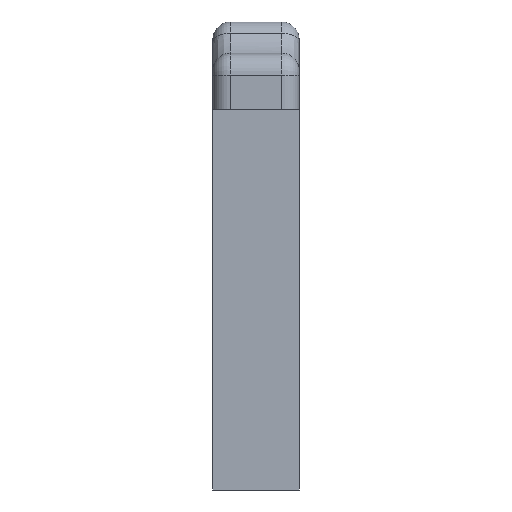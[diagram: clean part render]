
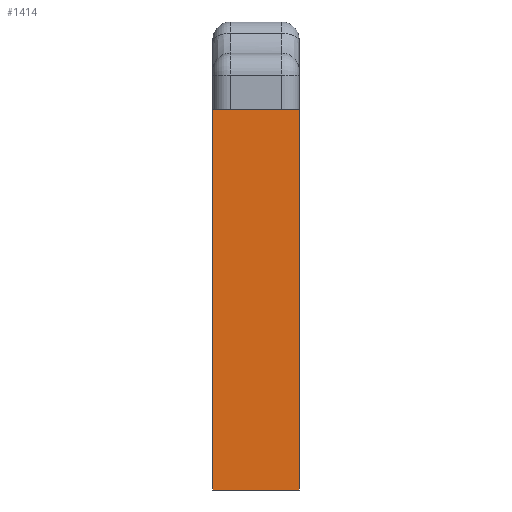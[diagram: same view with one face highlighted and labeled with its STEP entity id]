
A CAD part, front view. The second image highlights one B-rep face of the part: STEP entity #1414.
In plain terms, the highlighted planar face has unit normal (0, -1, 0).
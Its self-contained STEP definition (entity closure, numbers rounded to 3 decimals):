
#30 = EDGE_CURVE ( 'NONE', #1601, #479, #509, .T. ) ;
#61 = DIRECTION ( 'NONE',  ( -1., 0., 0. ) ) ;
#64 = CARTESIAN_POINT ( 'NONE',  ( 9.898, -2.5, -38.75 ) ) ;
#127 = ORIENTED_EDGE ( 'NONE', *, *, #1538, .T. ) ;
#147 = CARTESIAN_POINT ( 'NONE',  ( 9.898, -2.5, 5. ) ) ;
#215 = DIRECTION ( 'NONE',  ( 0., 0., 1. ) ) ;
#233 = DIRECTION ( 'NONE',  ( 0., 1., 0. ) ) ;
#237 = CARTESIAN_POINT ( 'NONE',  ( 9.898, -2.5, 15. ) ) ;
#337 = PLANE ( 'NONE',  #654 ) ;
#467 = VECTOR ( 'NONE', #1634, 1000. ) ;
#479 = VERTEX_POINT ( 'NONE', #823 ) ;
#486 = LINE ( 'NONE', #537, #467 ) ;
#488 = VECTOR ( 'NONE', #1300, 1000. ) ;
#505 = DIRECTION ( 'NONE',  ( 1., 0., 0. ) ) ;
#509 = LINE ( 'NONE', #1474, #488 ) ;
#514 = CARTESIAN_POINT ( 'NONE',  ( 9.898, -2.5, 5. ) ) ;
#529 = VERTEX_POINT ( 'NONE', #739 ) ;
#537 = CARTESIAN_POINT ( 'NONE',  ( 0., -2.5, 15. ) ) ;
#616 = FACE_OUTER_BOUND ( 'NONE', #986, .T. ) ;
#654 = AXIS2_PLACEMENT_3D ( 'NONE', #237, #233, #215 ) ;
#739 = CARTESIAN_POINT ( 'NONE',  ( 0., -2.5, 5. ) ) ;
#823 = CARTESIAN_POINT ( 'NONE',  ( 9.898, -2.5, -38.75 ) ) ;
#885 = EDGE_CURVE ( 'NONE', #479, #1052, #1165, .T. ) ;
#935 = VECTOR ( 'NONE', #505, 1000. ) ;
#957 = ORIENTED_EDGE ( 'NONE', *, *, #1108, .F. ) ;
#958 = LINE ( 'NONE', #147, #935 ) ;
#986 = EDGE_LOOP ( 'NONE', ( #957, #127, #1262, #1286 ) ) ;
#1052 = VERTEX_POINT ( 'NONE', #1321 ) ;
#1108 = EDGE_CURVE ( 'NONE', #529, #1601, #958, .T. ) ;
#1165 = LINE ( 'NONE', #64, #1182 ) ;
#1182 = VECTOR ( 'NONE', #61, 1000. ) ;
#1262 = ORIENTED_EDGE ( 'NONE', *, *, #885, .F. ) ;
#1286 = ORIENTED_EDGE ( 'NONE', *, *, #30, .F. ) ;
#1300 = DIRECTION ( 'NONE',  ( 0., 0., -1. ) ) ;
#1321 = CARTESIAN_POINT ( 'NONE',  ( 0., -2.5, -38.75 ) ) ;
#1414 = ADVANCED_FACE ( 'NONE', ( #616 ), #337, .F. ) ;
#1474 = CARTESIAN_POINT ( 'NONE',  ( 9.898, -2.5, 15. ) ) ;
#1538 = EDGE_CURVE ( 'NONE', #529, #1052, #486, .T. ) ;
#1601 = VERTEX_POINT ( 'NONE', #514 ) ;
#1634 = DIRECTION ( 'NONE',  ( 0., 0., -1. ) ) ;
